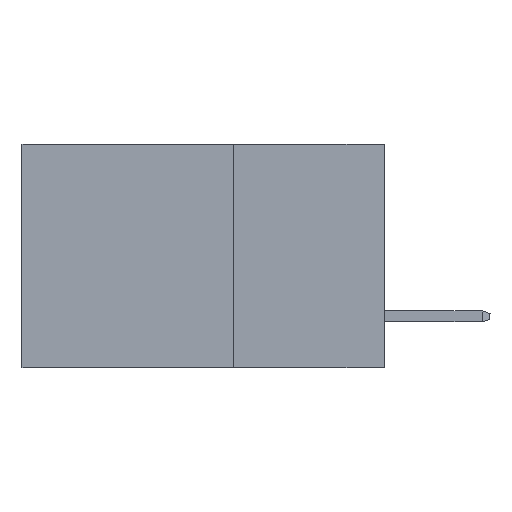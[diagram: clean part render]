
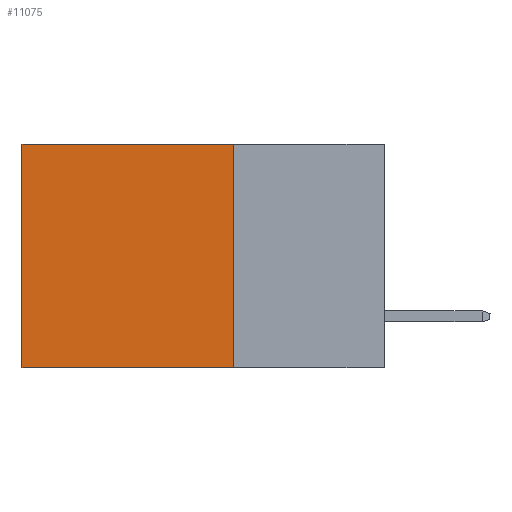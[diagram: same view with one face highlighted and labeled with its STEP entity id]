
A CAD part, left-side view. The second image highlights one B-rep face of the part: STEP entity #11075.
In plain terms, the highlighted planar face has unit normal (-1, 0, 0).
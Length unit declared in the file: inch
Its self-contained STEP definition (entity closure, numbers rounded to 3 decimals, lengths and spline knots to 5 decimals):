
#139 = DIRECTION ( 'NONE',  ( 0., 0., -1. ) ) ;
#949 = LINE ( 'NONE', #6291, #9044 ) ;
#1437 = CARTESIAN_POINT ( 'NONE',  ( 0.2615, 0.6, 0. ) ) ;
#1469 = AXIS2_PLACEMENT_3D ( 'NONE', #4195, #6929, #8630 ) ;
#1788 = CARTESIAN_POINT ( 'NONE',  ( 0.2615, 0.6, -0.37 ) ) ;
#2422 = EDGE_CURVE ( 'NONE', #8760, #9263, #2654, .T. ) ;
#2582 = CARTESIAN_POINT ( 'NONE',  ( 0.2615, 0.6, -0.37 ) ) ;
#2602 = ORIENTED_EDGE ( 'NONE', *, *, #6856, .F. ) ;
#2654 = LINE ( 'NONE', #4468, #10525 ) ;
#2974 = LINE ( 'NONE', #9878, #5545 ) ;
#3269 = ORIENTED_EDGE ( 'NONE', *, *, #10121, .T. ) ;
#3614 = VERTEX_POINT ( 'NONE', #1788 ) ;
#3661 = ORIENTED_EDGE ( 'NONE', *, *, #2422, .T. ) ;
#4195 = CARTESIAN_POINT ( 'NONE',  ( 0.2615, 0.25, -0.37 ) ) ;
#4468 = CARTESIAN_POINT ( 'NONE',  ( 0.2615, 0.25, 0. ) ) ;
#5514 = DIRECTION ( 'NONE',  ( 0., 1., 0. ) ) ;
#5545 = VECTOR ( 'NONE', #139, 39.37008 ) ;
#6124 = DIRECTION ( 'NONE',  ( 0., 1., 0. ) ) ;
#6291 = CARTESIAN_POINT ( 'NONE',  ( 0.2615, 0.25, -0.37 ) ) ;
#6854 = VERTEX_POINT ( 'NONE', #8856 ) ;
#6856 = EDGE_CURVE ( 'NONE', #6854, #3614, #949, .T. ) ;
#6929 = DIRECTION ( 'NONE',  ( 1., 0., 0. ) ) ;
#7992 = LINE ( 'NONE', #2582, #10581 ) ;
#8393 = EDGE_LOOP ( 'NONE', ( #3269, #2602, #10409, #3661 ) ) ;
#8630 = DIRECTION ( 'NONE',  ( 0., 0., -1. ) ) ;
#8760 = VERTEX_POINT ( 'NONE', #10837 ) ;
#8762 = DIRECTION ( 'NONE',  ( 0., 0., -1. ) ) ;
#8856 = CARTESIAN_POINT ( 'NONE',  ( 0.2615, 0.25, -0.37 ) ) ;
#9044 = VECTOR ( 'NONE', #6124, 39.37008 ) ;
#9263 = VERTEX_POINT ( 'NONE', #1437 ) ;
#9878 = CARTESIAN_POINT ( 'NONE',  ( 0.2615, 0.25, -0.37 ) ) ;
#10121 = EDGE_CURVE ( 'NONE', #9263, #3614, #7992, .T. ) ;
#10354 = EDGE_CURVE ( 'NONE', #8760, #6854, #2974, .T. ) ;
#10409 = ORIENTED_EDGE ( 'NONE', *, *, #10354, .F. ) ;
#10498 = FACE_OUTER_BOUND ( 'NONE', #8393, .T. ) ;
#10525 = VECTOR ( 'NONE', #5514, 39.37008 ) ;
#10555 = PLANE ( 'NONE',  #1469 ) ;
#10581 = VECTOR ( 'NONE', #8762, 39.37008 ) ;
#10837 = CARTESIAN_POINT ( 'NONE',  ( 0.2615, 0.25, 0. ) ) ;
#11075 = ADVANCED_FACE ( 'NONE', ( #10498 ), #10555, .F. ) ;
